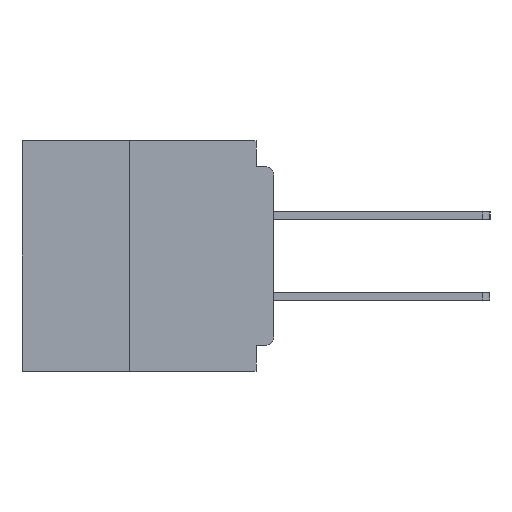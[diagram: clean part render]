
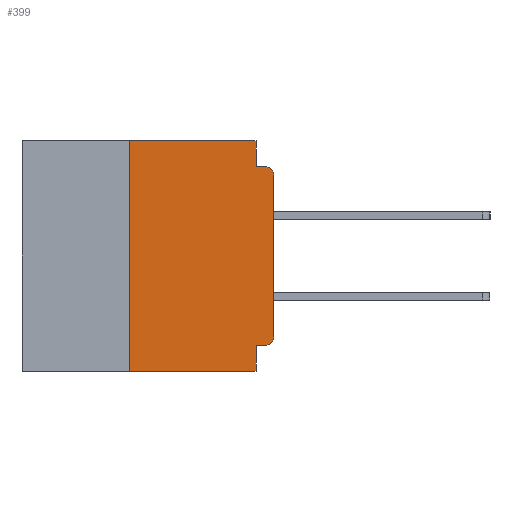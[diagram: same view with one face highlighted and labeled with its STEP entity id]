
A CAD part, left-side view. The second image highlights one B-rep face of the part: STEP entity #399.
In plain terms, the highlighted planar face has unit normal (-1, 0, 0).
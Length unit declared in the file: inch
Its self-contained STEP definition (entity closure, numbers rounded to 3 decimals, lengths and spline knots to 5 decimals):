
#64 = LINE ( 'NONE', #14246, #10940 ) ;
#399 = ADVANCED_FACE ( 'NONE', ( #39187 ), #31273, .F. ) ;
#771 = DIRECTION ( 'NONE',  ( 0., 0., -1. ) ) ;
#2031 = LINE ( 'NONE', #41761, #43515 ) ;
#2455 = CARTESIAN_POINT ( 'NONE',  ( 0., 0., -0.045 ) ) ;
#2869 = VERTEX_POINT ( 'NONE', #36173 ) ;
#2962 = VERTEX_POINT ( 'NONE', #31886 ) ;
#3991 = EDGE_CURVE ( 'NONE', #37714, #2869, #15228, .T. ) ;
#4565 = AXIS2_PLACEMENT_3D ( 'NONE', #5467, #33549, #9597 ) ;
#5428 = ORIENTED_EDGE ( 'NONE', *, *, #30676, .T. ) ;
#5467 = CARTESIAN_POINT ( 'NONE',  ( 0., 0.015, -0.06 ) ) ;
#5613 = DIRECTION ( 'NONE',  ( 0., -1., 0. ) ) ;
#6349 = VECTOR ( 'NONE', #25650, 39.37008 ) ;
#6934 = ORIENTED_EDGE ( 'NONE', *, *, #19400, .F. ) ;
#7074 = CARTESIAN_POINT ( 'NONE',  ( 0., 0.25, 0. ) ) ;
#7450 = ORIENTED_EDGE ( 'NONE', *, *, #11806, .F. ) ;
#7824 = VERTEX_POINT ( 'NONE', #38302 ) ;
#7965 = VERTEX_POINT ( 'NONE', #7074 ) ;
#8567 = VERTEX_POINT ( 'NONE', #34882 ) ;
#9597 = DIRECTION ( 'NONE',  ( 0., 0., -1. ) ) ;
#10706 = CARTESIAN_POINT ( 'NONE',  ( 0., 0.25, -0.4 ) ) ;
#10940 = VECTOR ( 'NONE', #42178, 39.37008 ) ;
#11806 = EDGE_CURVE ( 'NONE', #2962, #13968, #64, .T. ) ;
#12108 = CARTESIAN_POINT ( 'NONE',  ( 0., 0., -0.06 ) ) ;
#13968 = VERTEX_POINT ( 'NONE', #14408 ) ;
#14246 = CARTESIAN_POINT ( 'NONE',  ( 0., 0., -0.355 ) ) ;
#14408 = CARTESIAN_POINT ( 'NONE',  ( 0., 0.031, -0.355 ) ) ;
#14680 = CARTESIAN_POINT ( 'NONE',  ( 0., 0.437, 0. ) ) ;
#15085 = ORIENTED_EDGE ( 'NONE', *, *, #40410, .F. ) ;
#15228 = CIRCLE ( 'NONE', #4565, 0.015 ) ;
#15258 = CARTESIAN_POINT ( 'NONE',  ( 0., 0.437, 0. ) ) ;
#15986 = AXIS2_PLACEMENT_3D ( 'NONE', #48826, #25014, #771 ) ;
#16402 = EDGE_LOOP ( 'NONE', ( #37664, #25916, #6934, #21212, #43913, #25646, #5428, #15085, #7450, #21133 ) ) ;
#16926 = VECTOR ( 'NONE', #46653, 39.37008 ) ;
#17106 = LINE ( 'NONE', #45660, #6349 ) ;
#18376 = VERTEX_POINT ( 'NONE', #35948 ) ;
#19400 = EDGE_CURVE ( 'NONE', #8567, #2869, #38178, .T. ) ;
#20666 = CARTESIAN_POINT ( 'NONE',  ( 0., 0.031, -0.4 ) ) ;
#21133 = ORIENTED_EDGE ( 'NONE', *, *, #38518, .T. ) ;
#21212 = ORIENTED_EDGE ( 'NONE', *, *, #22389, .F. ) ;
#22389 = EDGE_CURVE ( 'NONE', #18376, #8567, #17106, .T. ) ;
#25014 = DIRECTION ( 'NONE',  ( -1., 0., 0. ) ) ;
#25646 = ORIENTED_EDGE ( 'NONE', *, *, #27543, .F. ) ;
#25650 = DIRECTION ( 'NONE',  ( 0., 0., -1. ) ) ;
#25916 = ORIENTED_EDGE ( 'NONE', *, *, #3991, .T. ) ;
#26895 = DIRECTION ( 'NONE',  ( 0., 0., -1. ) ) ;
#27004 = DIRECTION ( 'NONE',  ( 1., 0., 0. ) ) ;
#27353 = DIRECTION ( 'NONE',  ( 0., -1., 0. ) ) ;
#27543 = EDGE_CURVE ( 'NONE', #39326, #7965, #41194, .T. ) ;
#28459 = LINE ( 'NONE', #49523, #48380 ) ;
#29032 = VECTOR ( 'NONE', #45208, 39.37008 ) ;
#30371 = AXIS2_PLACEMENT_3D ( 'NONE', #14680, #27004, #26895 ) ;
#30676 = EDGE_CURVE ( 'NONE', #39326, #33851, #28459, .T. ) ;
#31273 = PLANE ( 'NONE',  #30371 ) ;
#31886 = CARTESIAN_POINT ( 'NONE',  ( 0., 0.015, -0.355 ) ) ;
#33549 = DIRECTION ( 'NONE',  ( -1., 0., 0. ) ) ;
#33851 = VERTEX_POINT ( 'NONE', #20666 ) ;
#34882 = CARTESIAN_POINT ( 'NONE',  ( 0., 0.031, -0.045 ) ) ;
#35948 = CARTESIAN_POINT ( 'NONE',  ( 0., 0.031, 0. ) ) ;
#36173 = CARTESIAN_POINT ( 'NONE',  ( 0., 0.015, -0.045 ) ) ;
#37664 = ORIENTED_EDGE ( 'NONE', *, *, #45218, .T. ) ;
#37714 = VERTEX_POINT ( 'NONE', #12108 ) ;
#38178 = LINE ( 'NONE', #2455, #16926 ) ;
#38302 = CARTESIAN_POINT ( 'NONE',  ( 0., 0., -0.34 ) ) ;
#38518 = EDGE_CURVE ( 'NONE', #2962, #7824, #49750, .T. ) ;
#38890 = VECTOR ( 'NONE', #27353, 39.37008 ) ;
#38926 = CARTESIAN_POINT ( 'NONE',  ( 0., 0.25, -0.4 ) ) ;
#39187 = FACE_OUTER_BOUND ( 'NONE', #16402, .T. ) ;
#39326 = VERTEX_POINT ( 'NONE', #10706 ) ;
#40410 = EDGE_CURVE ( 'NONE', #13968, #33851, #42138, .T. ) ;
#41194 = LINE ( 'NONE', #38926, #50450 ) ;
#41761 = CARTESIAN_POINT ( 'NONE',  ( 0., 0., 0. ) ) ;
#42138 = LINE ( 'NONE', #49157, #29032 ) ;
#42161 = EDGE_CURVE ( 'NONE', #7965, #18376, #49421, .T. ) ;
#42178 = DIRECTION ( 'NONE',  ( 0., 1., 0. ) ) ;
#43105 = DIRECTION ( 'NONE',  ( 0., 0., 1. ) ) ;
#43515 = VECTOR ( 'NONE', #45926, 39.37008 ) ;
#43913 = ORIENTED_EDGE ( 'NONE', *, *, #42161, .F. ) ;
#45208 = DIRECTION ( 'NONE',  ( 0., 0., -1. ) ) ;
#45218 = EDGE_CURVE ( 'NONE', #7824, #37714, #2031, .T. ) ;
#45660 = CARTESIAN_POINT ( 'NONE',  ( 0., 0.031, 0. ) ) ;
#45926 = DIRECTION ( 'NONE',  ( 0., 0., 1. ) ) ;
#46653 = DIRECTION ( 'NONE',  ( 0., -1., 0. ) ) ;
#48380 = VECTOR ( 'NONE', #5613, 39.37008 ) ;
#48826 = CARTESIAN_POINT ( 'NONE',  ( 0., 0.015, -0.34 ) ) ;
#49157 = CARTESIAN_POINT ( 'NONE',  ( 0., 0.031, -0.4 ) ) ;
#49421 = LINE ( 'NONE', #15258, #38890 ) ;
#49523 = CARTESIAN_POINT ( 'NONE',  ( 0., 0.437, -0.4 ) ) ;
#49750 = CIRCLE ( 'NONE', #15986, 0.015 ) ;
#50450 = VECTOR ( 'NONE', #43105, 39.37008 ) ;
